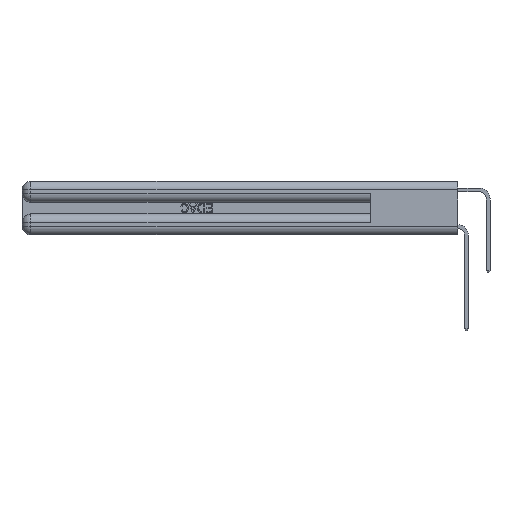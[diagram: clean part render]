
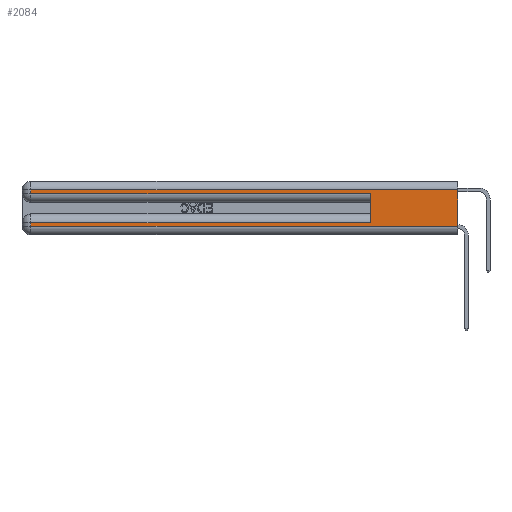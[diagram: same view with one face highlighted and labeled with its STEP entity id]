
A CAD part, left-side view. The second image highlights one B-rep face of the part: STEP entity #2084.
In plain terms, the highlighted planar face has unit normal (-1, 0, 0).
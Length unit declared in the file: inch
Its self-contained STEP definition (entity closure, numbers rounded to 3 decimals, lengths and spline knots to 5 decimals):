
#215 = EDGE_CURVE ( 'NONE', #28578, #24585, #27084, .T. ) ;
#653 = ORIENTED_EDGE ( 'NONE', *, *, #3390, .T. ) ;
#1565 = CARTESIAN_POINT ( 'NONE',  ( 0., 0., 0.37 ) ) ;
#1714 = PLANE ( 'NONE',  #10964 ) ;
#2084 = ADVANCED_FACE ( 'NONE', ( #15898 ), #1714, .F. ) ;
#2238 = ORIENTED_EDGE ( 'NONE', *, *, #13883, .F. ) ;
#2452 = VERTEX_POINT ( 'NONE', #20035 ) ;
#3200 = LINE ( 'NONE', #5646, #7758 ) ;
#3390 = EDGE_CURVE ( 'NONE', #17506, #29307, #4239, .T. ) ;
#4160 = EDGE_CURVE ( 'NONE', #27924, #10088, #13564, .T. ) ;
#4239 = LINE ( 'NONE', #27752, #13415 ) ;
#4437 = ORIENTED_EDGE ( 'NONE', *, *, #215, .T. ) ;
#4461 = EDGE_CURVE ( 'NONE', #9422, #28578, #3200, .T. ) ;
#4599 = VECTOR ( 'NONE', #9835, 39.37008 ) ;
#4898 = CARTESIAN_POINT ( 'NONE',  ( 0., 0.6, 0.085 ) ) ;
#5351 = VECTOR ( 'NONE', #24106, 39.37008 ) ;
#5646 = CARTESIAN_POINT ( 'NONE',  ( 0., 2.94, 0.37 ) ) ;
#6602 = DIRECTION ( 'NONE',  ( 1., 0., 0. ) ) ;
#7401 = DIRECTION ( 'NONE',  ( 0., -1., 0. ) ) ;
#7436 = VECTOR ( 'NONE', #8779, 39.37008 ) ;
#7758 = VECTOR ( 'NONE', #14924, 39.37008 ) ;
#8779 = DIRECTION ( 'NONE',  ( 0., 1., 0. ) ) ;
#9422 = VERTEX_POINT ( 'NONE', #18203 ) ;
#9679 = EDGE_LOOP ( 'NONE', ( #2238, #23386, #653, #17166, #17063, #13643, #27195, #4437 ) ) ;
#9702 = VECTOR ( 'NONE', #29644, 39.37008 ) ;
#9704 = LINE ( 'NONE', #28327, #26251 ) ;
#9798 = CARTESIAN_POINT ( 'NONE',  ( 0., 0.6, 0.285 ) ) ;
#9835 = DIRECTION ( 'NONE',  ( 0., 0., -1. ) ) ;
#10088 = VERTEX_POINT ( 'NONE', #9798 ) ;
#10964 = AXIS2_PLACEMENT_3D ( 'NONE', #1565, #6602, #29819 ) ;
#11434 = CARTESIAN_POINT ( 'NONE',  ( 0., 2.94, 0.31 ) ) ;
#11940 = CARTESIAN_POINT ( 'NONE',  ( 0., 0., 0.06 ) ) ;
#13316 = CARTESIAN_POINT ( 'NONE',  ( 0., 0., 0.085 ) ) ;
#13415 = VECTOR ( 'NONE', #16283, 39.37008 ) ;
#13564 = LINE ( 'NONE', #29494, #9702 ) ;
#13643 = ORIENTED_EDGE ( 'NONE', *, *, #16521, .T. ) ;
#13883 = EDGE_CURVE ( 'NONE', #2452, #24585, #24136, .T. ) ;
#14682 = CARTESIAN_POINT ( 'NONE',  ( 0., 0., 0.37 ) ) ;
#14924 = DIRECTION ( 'NONE',  ( 0., 0., -1. ) ) ;
#15331 = CARTESIAN_POINT ( 'NONE',  ( 0., 2.94, 0.06 ) ) ;
#15898 = FACE_OUTER_BOUND ( 'NONE', #9679, .T. ) ;
#16283 = DIRECTION ( 'NONE',  ( 0., 0., -1. ) ) ;
#16521 = EDGE_CURVE ( 'NONE', #27924, #9422, #29998, .T. ) ;
#17063 = ORIENTED_EDGE ( 'NONE', *, *, #4160, .F. ) ;
#17166 = ORIENTED_EDGE ( 'NONE', *, *, #21917, .T. ) ;
#17506 = VERTEX_POINT ( 'NONE', #11434 ) ;
#18203 = CARTESIAN_POINT ( 'NONE',  ( 0., 2.94, 0.085 ) ) ;
#18340 = VECTOR ( 'NONE', #20519, 39.37008 ) ;
#19529 = CARTESIAN_POINT ( 'NONE',  ( 0., 2.94, 0.285 ) ) ;
#20035 = CARTESIAN_POINT ( 'NONE',  ( 0., 0., 0.31 ) ) ;
#20519 = DIRECTION ( 'NONE',  ( 0., -1., 0. ) ) ;
#21917 = EDGE_CURVE ( 'NONE', #29307, #10088, #9704, .T. ) ;
#22836 = EDGE_CURVE ( 'NONE', #2452, #17506, #28426, .T. ) ;
#23386 = ORIENTED_EDGE ( 'NONE', *, *, #22836, .T. ) ;
#24106 = DIRECTION ( 'NONE',  ( 0., 1., 0. ) ) ;
#24136 = LINE ( 'NONE', #14682, #4599 ) ;
#24585 = VERTEX_POINT ( 'NONE', #11940 ) ;
#24922 = CARTESIAN_POINT ( 'NONE',  ( 0., 0., 0.06 ) ) ;
#26251 = VECTOR ( 'NONE', #7401, 39.37008 ) ;
#26270 = CARTESIAN_POINT ( 'NONE',  ( 0., 0., 0.31 ) ) ;
#27084 = LINE ( 'NONE', #24922, #18340 ) ;
#27195 = ORIENTED_EDGE ( 'NONE', *, *, #4461, .T. ) ;
#27752 = CARTESIAN_POINT ( 'NONE',  ( 0., 2.94, 0.37 ) ) ;
#27924 = VERTEX_POINT ( 'NONE', #4898 ) ;
#28327 = CARTESIAN_POINT ( 'NONE',  ( 0., 0., 0.285 ) ) ;
#28426 = LINE ( 'NONE', #26270, #5351 ) ;
#28578 = VERTEX_POINT ( 'NONE', #15331 ) ;
#29307 = VERTEX_POINT ( 'NONE', #19529 ) ;
#29494 = CARTESIAN_POINT ( 'NONE',  ( 0., 0.6, 0.145 ) ) ;
#29644 = DIRECTION ( 'NONE',  ( 0., 0., 1. ) ) ;
#29819 = DIRECTION ( 'NONE',  ( 0., 0., -1. ) ) ;
#29998 = LINE ( 'NONE', #13316, #7436 ) ;
